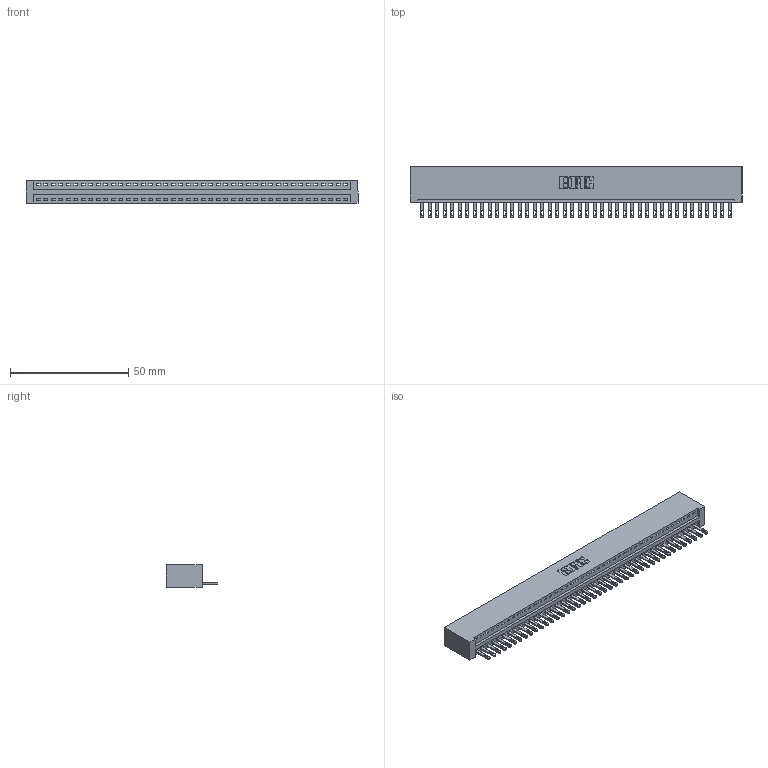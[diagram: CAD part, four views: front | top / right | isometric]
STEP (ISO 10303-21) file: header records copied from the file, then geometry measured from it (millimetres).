
FILE_DESCRIPTION (( 'STEP AP203' ), '1' );
FILE_NAME ('346-042-500-101.STEP', '2022-05-09T13:52:45', ( '' ), ( '' ), 'SwSTEP 2.0', 'SolidWorks 2020', '' );
FILE_SCHEMA (( 'CONFIG_CONTROL_DESIGN' ));
Length unit declared in the file: inch
Products named in the file (3): 345-292-001_345-293-100; 346-042-500-101; 346 Part_No Mounting Lugs
Assembly tree (43 placements, depth 2):
  346-042-500-101
    346 Part_No Mounting Lugs
    345-292-001_345-293-100  x42
Bounding box: 140.59 x 21.84 x 9.4 mm (x, y, z)
Volume: 14032.9 mm3; surface area: 17712.3 mm2
Topology: 43 solids, 43 shells, 2382 faces, 7361 edges, 4906 vertices
Faces by surface type: plane 1500, cylinder 882
Entity records: 25719 total; most frequent: CARTESIAN_POINT 4414, ORIENTED_EDGE 4390, DIRECTION 3891, EDGE_CURVE 2195, VECTOR 1899, LINE 1899, VERTEX_POINT 1462, AXIS2_PLACEMENT_3D 996
